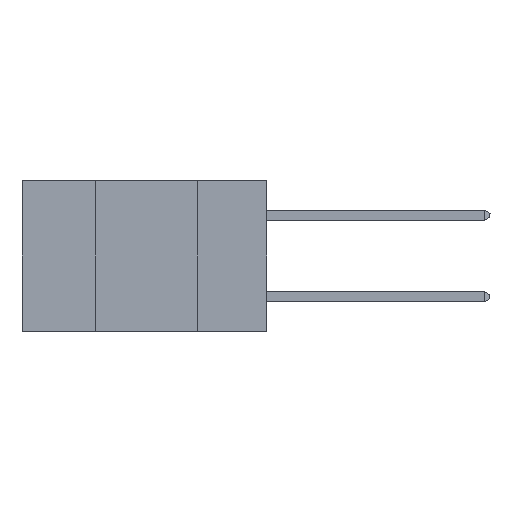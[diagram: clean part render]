
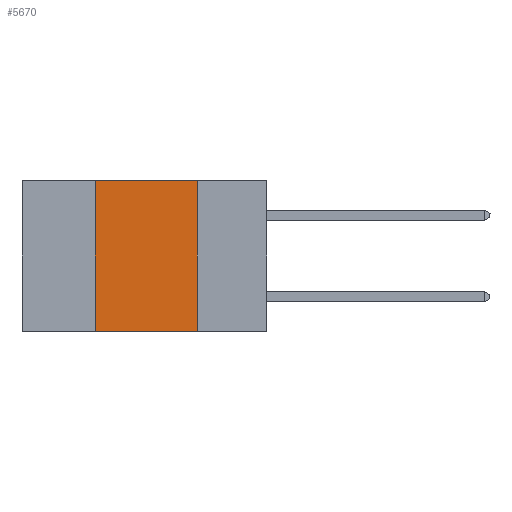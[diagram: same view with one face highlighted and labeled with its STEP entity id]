
A CAD part, left-side view. The second image highlights one B-rep face of the part: STEP entity #5670.
In plain terms, the highlighted planar face has unit normal (-1, 0, 0).
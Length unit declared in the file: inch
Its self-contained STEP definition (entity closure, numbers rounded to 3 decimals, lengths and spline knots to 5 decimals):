
#121 = CARTESIAN_POINT ( 'NONE',  ( 0., 0.17, -0.37 ) ) ;
#639 = FACE_OUTER_BOUND ( 'NONE', #22942, .T. ) ;
#850 = ORIENTED_EDGE ( 'NONE', *, *, #6079, .T. ) ;
#1453 = VECTOR ( 'NONE', #17315, 39.37008 ) ;
#1698 = EDGE_CURVE ( 'NONE', #17798, #21791, #2015, .T. ) ;
#2015 = LINE ( 'NONE', #3926, #3219 ) ;
#3104 = DIRECTION ( 'NONE',  ( 0., 0., -1. ) ) ;
#3219 = VECTOR ( 'NONE', #16577, 39.37008 ) ;
#3926 = CARTESIAN_POINT ( 'NONE',  ( 0., 0.42, 0. ) ) ;
#4765 = ORIENTED_EDGE ( 'NONE', *, *, #1698, .F. ) ;
#5123 = VERTEX_POINT ( 'NONE', #18011 ) ;
#5670 = ADVANCED_FACE ( 'NONE', ( #639 ), #19044, .F. ) ;
#6079 = EDGE_CURVE ( 'NONE', #17798, #18856, #15402, .T. ) ;
#6337 = VECTOR ( 'NONE', #18562, 39.37008 ) ;
#7513 = CARTESIAN_POINT ( 'NONE',  ( 0., 0.6, 0. ) ) ;
#7618 = LINE ( 'NONE', #7513, #6337 ) ;
#8062 = ORIENTED_EDGE ( 'NONE', *, *, #20403, .F. ) ;
#10033 = DIRECTION ( 'NONE',  ( 1., 0., 0. ) ) ;
#12069 = VECTOR ( 'NONE', #3104, 39.37008 ) ;
#12368 = CARTESIAN_POINT ( 'NONE',  ( 0., 0.17, 0. ) ) ;
#15402 = LINE ( 'NONE', #19023, #1453 ) ;
#15655 = DIRECTION ( 'NONE',  ( 0., 0., -1. ) ) ;
#15730 = LINE ( 'NONE', #12368, #12069 ) ;
#16577 = DIRECTION ( 'NONE',  ( 0., 0., 1. ) ) ;
#17315 = DIRECTION ( 'NONE',  ( 0., -1., 0. ) ) ;
#17798 = VERTEX_POINT ( 'NONE', #21285 ) ;
#18011 = CARTESIAN_POINT ( 'NONE',  ( 0., 0.17, 0. ) ) ;
#18562 = DIRECTION ( 'NONE',  ( 0., -1., 0. ) ) ;
#18856 = VERTEX_POINT ( 'NONE', #121 ) ;
#19023 = CARTESIAN_POINT ( 'NONE',  ( 0., 0.6, -0.37 ) ) ;
#19044 = PLANE ( 'NONE',  #20643 ) ;
#19086 = EDGE_CURVE ( 'NONE', #5123, #18856, #15730, .T. ) ;
#19922 = ORIENTED_EDGE ( 'NONE', *, *, #19086, .F. ) ;
#20403 = EDGE_CURVE ( 'NONE', #21791, #5123, #7618, .T. ) ;
#20643 = AXIS2_PLACEMENT_3D ( 'NONE', #22792, #10033, #15655 ) ;
#21285 = CARTESIAN_POINT ( 'NONE',  ( 0., 0.42, -0.37 ) ) ;
#21791 = VERTEX_POINT ( 'NONE', #22165 ) ;
#22165 = CARTESIAN_POINT ( 'NONE',  ( 0., 0.42, 0. ) ) ;
#22792 = CARTESIAN_POINT ( 'NONE',  ( 0., 0.6, 0. ) ) ;
#22942 = EDGE_LOOP ( 'NONE', ( #19922, #8062, #4765, #850 ) ) ;
